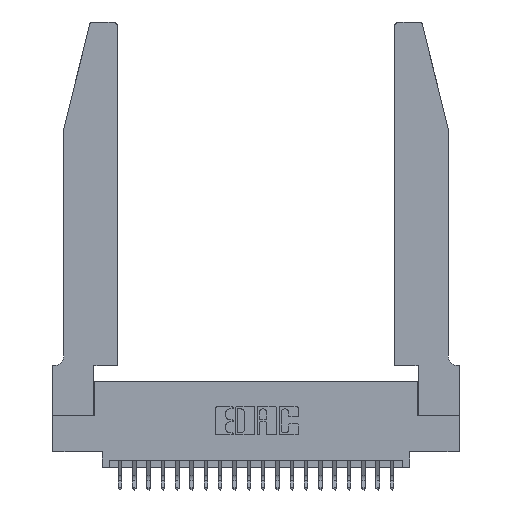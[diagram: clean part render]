
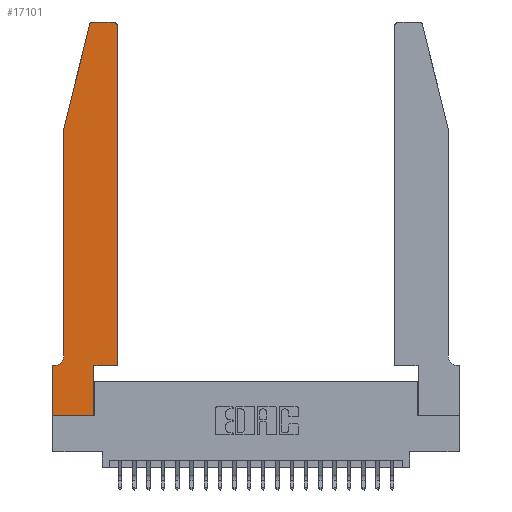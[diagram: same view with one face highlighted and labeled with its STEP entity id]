
A CAD part, top view. The second image highlights one B-rep face of the part: STEP entity #17101.
In plain terms, the highlighted planar face has unit normal (0, 0, 1).
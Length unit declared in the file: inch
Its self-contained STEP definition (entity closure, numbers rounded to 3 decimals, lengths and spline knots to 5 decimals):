
#17 = EDGE_CURVE ( 'NONE', #14513, #13187, #20170, .T. ) ;
#559 = DIRECTION ( 'NONE',  ( 1., 0., 0. ) ) ;
#619 = VECTOR ( 'NONE', #21639, 39.37008 ) ;
#734 = CARTESIAN_POINT ( 'NONE',  ( 0.4505, 0.35, 0.37 ) ) ;
#1228 = VECTOR ( 'NONE', #4442, 39.37008 ) ;
#1496 = LINE ( 'NONE', #734, #1228 ) ;
#1898 = DIRECTION ( 'NONE',  ( -0.239, -0.971, 0. ) ) ;
#2323 = DIRECTION ( 'NONE',  ( -1., 0., 0. ) ) ;
#2391 = CARTESIAN_POINT ( 'NONE',  ( 0.4505, 2.72, 0.37 ) ) ;
#2411 = ORIENTED_EDGE ( 'NONE', *, *, #4650, .T. ) ;
#2717 = DIRECTION ( 'NONE',  ( 1., 0., 0. ) ) ;
#3049 = AXIS2_PLACEMENT_3D ( 'NONE', #13434, #4349, #2717 ) ;
#3275 = VERTEX_POINT ( 'NONE', #14172 ) ;
#3538 = VERTEX_POINT ( 'NONE', #22603 ) ;
#3557 = EDGE_LOOP ( 'NONE', ( #16412, #7410, #5381, #5341, #23370, #2411, #9232, #7819, #7546, #18485, #15097, #17967 ) ) ;
#3962 = CARTESIAN_POINT ( 'NONE',  ( 0., 0., 0.37 ) ) ;
#4349 = DIRECTION ( 'NONE',  ( 0., 0., 1. ) ) ;
#4442 = DIRECTION ( 'NONE',  ( 0., 1., 0. ) ) ;
#4650 = EDGE_CURVE ( 'NONE', #22828, #5943, #5586, .T. ) ;
#4910 = LINE ( 'NONE', #18177, #20703 ) ;
#5047 = EDGE_CURVE ( 'NONE', #13187, #18186, #10761, .T. ) ;
#5111 = CARTESIAN_POINT ( 'NONE',  ( 0.2865, 0.35, 0.37 ) ) ;
#5341 = ORIENTED_EDGE ( 'NONE', *, *, #10671, .T. ) ;
#5381 = ORIENTED_EDGE ( 'NONE', *, *, #10563, .T. ) ;
#5586 = LINE ( 'NONE', #22415, #22539 ) ;
#5610 = CIRCLE ( 'NONE', #16069, 0.07 ) ;
#5943 = VERTEX_POINT ( 'NONE', #11020 ) ;
#6421 = CARTESIAN_POINT ( 'NONE',  ( 0.0055, 0.35, 0.37 ) ) ;
#6491 = CARTESIAN_POINT ( 'NONE',  ( 0., 0., 0.37 ) ) ;
#6575 = CARTESIAN_POINT ( 'NONE',  ( 0.4505, 0.35, 0.37 ) ) ;
#7119 = VECTOR ( 'NONE', #19349, 39.37008 ) ;
#7410 = ORIENTED_EDGE ( 'NONE', *, *, #5047, .T. ) ;
#7426 = VECTOR ( 'NONE', #17415, 39.37008 ) ;
#7442 = CARTESIAN_POINT ( 'NONE',  ( 0.4205, 2.72, 0.37 ) ) ;
#7546 = ORIENTED_EDGE ( 'NONE', *, *, #23361, .T. ) ;
#7819 = ORIENTED_EDGE ( 'NONE', *, *, #9937, .T. ) ;
#7886 = DIRECTION ( 'NONE',  ( 0., 0., 1. ) ) ;
#8270 = VERTEX_POINT ( 'NONE', #17676 ) ;
#8516 = FACE_OUTER_BOUND ( 'NONE', #3557, .T. ) ;
#9232 = ORIENTED_EDGE ( 'NONE', *, *, #12737, .T. ) ;
#9374 = EDGE_CURVE ( 'NONE', #3538, #18692, #17772, .T. ) ;
#9548 = CARTESIAN_POINT ( 'NONE',  ( 0.0755, 2., 0.37 ) ) ;
#9784 = CARTESIAN_POINT ( 'NONE',  ( 0.4505, 0.35, 0.37 ) ) ;
#9937 = EDGE_CURVE ( 'NONE', #19658, #20623, #19185, .T. ) ;
#10133 = AXIS2_PLACEMENT_3D ( 'NONE', #17028, #7886, #559 ) ;
#10563 = EDGE_CURVE ( 'NONE', #18186, #8270, #22953, .T. ) ;
#10671 = EDGE_CURVE ( 'NONE', #8270, #3275, #4910, .T. ) ;
#10761 = CIRCLE ( 'NONE', #10133, 0.03 ) ;
#10784 = EDGE_CURVE ( 'NONE', #3275, #22828, #5610, .T. ) ;
#11020 = CARTESIAN_POINT ( 'NONE',  ( 0., 0.35, 0.37 ) ) ;
#12152 = EDGE_CURVE ( 'NONE', #18692, #12571, #1496, .T. ) ;
#12571 = VERTEX_POINT ( 'NONE', #2391 ) ;
#12628 = VECTOR ( 'NONE', #1898, 39.37008 ) ;
#12641 = DIRECTION ( 'NONE',  ( 0., -1., 0. ) ) ;
#12737 = EDGE_CURVE ( 'NONE', #5943, #19658, #14147, .T. ) ;
#12990 = DIRECTION ( 'NONE',  ( 1., 0., 0. ) ) ;
#13187 = VERTEX_POINT ( 'NONE', #21745 ) ;
#13395 = CIRCLE ( 'NONE', #19703, 0.03 ) ;
#13434 = CARTESIAN_POINT ( 'NONE',  ( 0., 0.35, 0.37 ) ) ;
#13745 = DIRECTION ( 'NONE',  ( 0., 0., -1. ) ) ;
#14147 = LINE ( 'NONE', #19820, #619 ) ;
#14172 = CARTESIAN_POINT ( 'NONE',  ( 0.0755, 0.42, 0.37 ) ) ;
#14513 = VERTEX_POINT ( 'NONE', #18882 ) ;
#14630 = CARTESIAN_POINT ( 'NONE',  ( 0.2605, 2.75, 0.37 ) ) ;
#15097 = ORIENTED_EDGE ( 'NONE', *, *, #12152, .T. ) ;
#15299 = PLANE ( 'NONE',  #3049 ) ;
#15548 = VECTOR ( 'NONE', #21936, 39.37008 ) ;
#15989 = LINE ( 'NONE', #5111, #21431 ) ;
#16069 = AXIS2_PLACEMENT_3D ( 'NONE', #18970, #13745, #22868 ) ;
#16412 = ORIENTED_EDGE ( 'NONE', *, *, #17, .T. ) ;
#16499 = DIRECTION ( 'NONE',  ( 0., 0., 1. ) ) ;
#17028 = CARTESIAN_POINT ( 'NONE',  ( 0.284, 2.72, 0.37 ) ) ;
#17101 = ADVANCED_FACE ( 'NONE', ( #8516 ), #15299, .T. ) ;
#17415 = DIRECTION ( 'NONE',  ( 1., 0., 0. ) ) ;
#17676 = CARTESIAN_POINT ( 'NONE',  ( 0.0755, 2., 0.37 ) ) ;
#17772 = LINE ( 'NONE', #6575, #7426 ) ;
#17956 = DIRECTION ( 'NONE',  ( 0., 1., 0. ) ) ;
#17967 = ORIENTED_EDGE ( 'NONE', *, *, #18134, .T. ) ;
#18134 = EDGE_CURVE ( 'NONE', #12571, #14513, #13395, .T. ) ;
#18177 = CARTESIAN_POINT ( 'NONE',  ( 0.0755, 2., 0.37 ) ) ;
#18186 = VERTEX_POINT ( 'NONE', #19136 ) ;
#18485 = ORIENTED_EDGE ( 'NONE', *, *, #9374, .T. ) ;
#18692 = VERTEX_POINT ( 'NONE', #9784 ) ;
#18882 = CARTESIAN_POINT ( 'NONE',  ( 0.4205, 2.75, 0.37 ) ) ;
#18970 = CARTESIAN_POINT ( 'NONE',  ( 0.0055, 0.42, 0.37 ) ) ;
#19136 = CARTESIAN_POINT ( 'NONE',  ( 0.25487, 2.72718, 0.37 ) ) ;
#19185 = LINE ( 'NONE', #6491, #7119 ) ;
#19349 = DIRECTION ( 'NONE',  ( 1., 0., 0. ) ) ;
#19652 = CARTESIAN_POINT ( 'NONE',  ( 0.2865, 0., 0.37 ) ) ;
#19658 = VERTEX_POINT ( 'NONE', #3962 ) ;
#19703 = AXIS2_PLACEMENT_3D ( 'NONE', #7442, #16499, #12990 ) ;
#19820 = CARTESIAN_POINT ( 'NONE',  ( 0., 0., 0.37 ) ) ;
#20170 = LINE ( 'NONE', #14630, #15548 ) ;
#20623 = VERTEX_POINT ( 'NONE', #19652 ) ;
#20703 = VECTOR ( 'NONE', #12641, 39.37008 ) ;
#21431 = VECTOR ( 'NONE', #17956, 39.37008 ) ;
#21639 = DIRECTION ( 'NONE',  ( 0., -1., 0. ) ) ;
#21745 = CARTESIAN_POINT ( 'NONE',  ( 0.284, 2.75, 0.37 ) ) ;
#21936 = DIRECTION ( 'NONE',  ( -1., 0., 0. ) ) ;
#22415 = CARTESIAN_POINT ( 'NONE',  ( 0.0755, 0.35, 0.37 ) ) ;
#22539 = VECTOR ( 'NONE', #2323, 39.37008 ) ;
#22603 = CARTESIAN_POINT ( 'NONE',  ( 0.2865, 0.35, 0.37 ) ) ;
#22828 = VERTEX_POINT ( 'NONE', #6421 ) ;
#22868 = DIRECTION ( 'NONE',  ( -1., 0., 0. ) ) ;
#22953 = LINE ( 'NONE', #9548, #12628 ) ;
#23361 = EDGE_CURVE ( 'NONE', #20623, #3538, #15989, .T. ) ;
#23370 = ORIENTED_EDGE ( 'NONE', *, *, #10784, .T. ) ;
